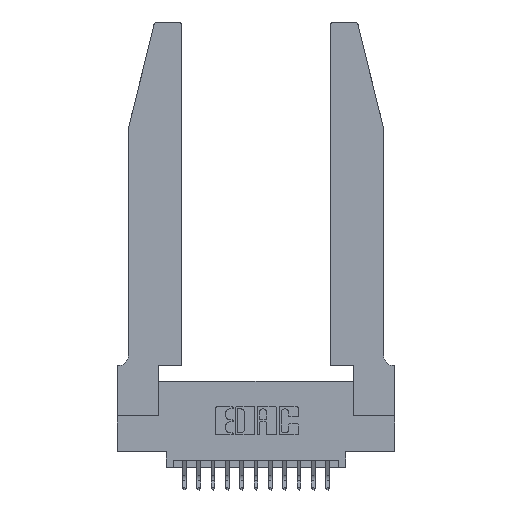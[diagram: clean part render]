
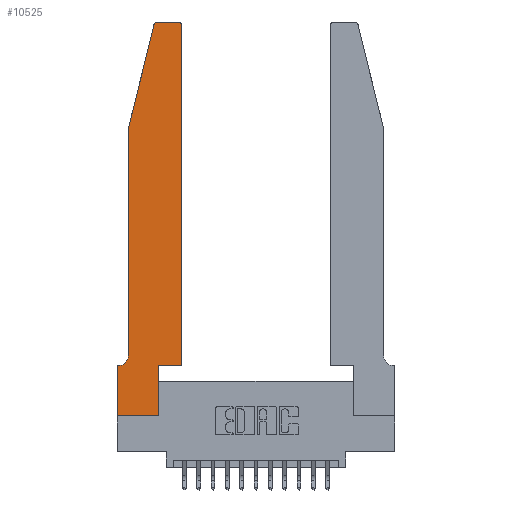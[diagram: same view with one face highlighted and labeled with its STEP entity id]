
A CAD part, top view. The second image highlights one B-rep face of the part: STEP entity #10525.
In plain terms, the highlighted planar face has unit normal (0, 0, 1).
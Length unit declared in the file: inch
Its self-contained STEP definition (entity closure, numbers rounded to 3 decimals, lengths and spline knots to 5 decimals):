
#69 = VERTEX_POINT ( 'NONE', #10907 ) ;
#88 = CARTESIAN_POINT ( 'NONE',  ( 0.2865, 0.35, 0.37 ) ) ;
#146 = VERTEX_POINT ( 'NONE', #14226 ) ;
#669 = ORIENTED_EDGE ( 'NONE', *, *, #8839, .T. ) ;
#888 = VERTEX_POINT ( 'NONE', #4528 ) ;
#901 = VECTOR ( 'NONE', #5757, 39.37008 ) ;
#990 = LINE ( 'NONE', #12985, #11191 ) ;
#1097 = CARTESIAN_POINT ( 'NONE',  ( 0.0755, 2., 0.37 ) ) ;
#1252 = VERTEX_POINT ( 'NONE', #10823 ) ;
#1785 = ORIENTED_EDGE ( 'NONE', *, *, #10338, .T. ) ;
#1799 = CARTESIAN_POINT ( 'NONE',  ( 0.4505, 0.35, 0.37 ) ) ;
#1834 = DIRECTION ( 'NONE',  ( -0.239, -0.971, 0. ) ) ;
#1997 = AXIS2_PLACEMENT_3D ( 'NONE', #11527, #16933, #4441 ) ;
#2156 = VERTEX_POINT ( 'NONE', #88 ) ;
#2163 = CIRCLE ( 'NONE', #17287, 0.03 ) ;
#2336 = CIRCLE ( 'NONE', #3263, 0.03 ) ;
#2740 = VERTEX_POINT ( 'NONE', #17051 ) ;
#2990 = VERTEX_POINT ( 'NONE', #9995 ) ;
#3242 = CARTESIAN_POINT ( 'NONE',  ( 0.4205, 2.72, 0.37 ) ) ;
#3263 = AXIS2_PLACEMENT_3D ( 'NONE', #3242, #10271, #14206 ) ;
#3358 = EDGE_CURVE ( 'NONE', #2156, #6280, #3509, .T. ) ;
#3509 = LINE ( 'NONE', #16581, #901 ) ;
#3695 = VECTOR ( 'NONE', #15009, 39.37008 ) ;
#3942 = LINE ( 'NONE', #11703, #5666 ) ;
#4131 = VECTOR ( 'NONE', #14072, 39.37008 ) ;
#4154 = VERTEX_POINT ( 'NONE', #14728 ) ;
#4338 = EDGE_CURVE ( 'NONE', #12381, #4154, #16650, .T. ) ;
#4441 = DIRECTION ( 'NONE',  ( 1., 0., 0. ) ) ;
#4528 = CARTESIAN_POINT ( 'NONE',  ( 0.4505, 2.72, 0.37 ) ) ;
#4531 = ORIENTED_EDGE ( 'NONE', *, *, #3358, .T. ) ;
#4559 = VECTOR ( 'NONE', #6593, 39.37008 ) ;
#4934 = FACE_OUTER_BOUND ( 'NONE', #13743, .T. ) ;
#5195 = DIRECTION ( 'NONE',  ( 1., 0., 0. ) ) ;
#5666 = VECTOR ( 'NONE', #7370, 39.37008 ) ;
#5748 = VERTEX_POINT ( 'NONE', #17686 ) ;
#5757 = DIRECTION ( 'NONE',  ( 1., 0., 0. ) ) ;
#5885 = VECTOR ( 'NONE', #16787, 39.37008 ) ;
#5897 = CARTESIAN_POINT ( 'NONE',  ( 0., 0., 0.37 ) ) ;
#6048 = ORIENTED_EDGE ( 'NONE', *, *, #14073, .T. ) ;
#6151 = ORIENTED_EDGE ( 'NONE', *, *, #4338, .T. ) ;
#6232 = EDGE_CURVE ( 'NONE', #6280, #888, #11156, .T. ) ;
#6280 = VERTEX_POINT ( 'NONE', #1799 ) ;
#6593 = DIRECTION ( 'NONE',  ( -1., 0., 0. ) ) ;
#6713 = LINE ( 'NONE', #16643, #4131 ) ;
#6915 = LINE ( 'NONE', #12071, #4559 ) ;
#7370 = DIRECTION ( 'NONE',  ( 0., -1., 0. ) ) ;
#7428 = EDGE_CURVE ( 'NONE', #2990, #14704, #3942, .T. ) ;
#7448 = VECTOR ( 'NONE', #14444, 39.37008 ) ;
#8438 = LINE ( 'NONE', #1097, #3695 ) ;
#8839 = EDGE_CURVE ( 'NONE', #69, #2740, #6915, .T. ) ;
#9248 = ORIENTED_EDGE ( 'NONE', *, *, #6232, .T. ) ;
#9437 = ORIENTED_EDGE ( 'NONE', *, *, #16857, .T. ) ;
#9463 = DIRECTION ( 'NONE',  ( -1., 0., 0. ) ) ;
#9907 = LINE ( 'NONE', #15202, #17660 ) ;
#9995 = CARTESIAN_POINT ( 'NONE',  ( 0., 0.35, 0.37 ) ) ;
#10022 = EDGE_CURVE ( 'NONE', #888, #69, #2336, .T. ) ;
#10271 = DIRECTION ( 'NONE',  ( 0., 0., 1. ) ) ;
#10294 = ORIENTED_EDGE ( 'NONE', *, *, #13024, .T. ) ;
#10338 = EDGE_CURVE ( 'NONE', #5748, #2156, #9907, .T. ) ;
#10525 = ADVANCED_FACE ( 'NONE', ( #4934 ), #14184, .T. ) ;
#10802 = CARTESIAN_POINT ( 'NONE',  ( 0.0055, 0.42, 0.37 ) ) ;
#10823 = CARTESIAN_POINT ( 'NONE',  ( 0.0755, 2., 0.37 ) ) ;
#10907 = CARTESIAN_POINT ( 'NONE',  ( 0.4205, 2.75, 0.37 ) ) ;
#11156 = LINE ( 'NONE', #11497, #7448 ) ;
#11191 = VECTOR ( 'NONE', #1834, 39.37008 ) ;
#11497 = CARTESIAN_POINT ( 'NONE',  ( 0.4505, 0.35, 0.37 ) ) ;
#11527 = CARTESIAN_POINT ( 'NONE',  ( 0., 0.35, 0.37 ) ) ;
#11654 = AXIS2_PLACEMENT_3D ( 'NONE', #10802, #12273, #9463 ) ;
#11703 = CARTESIAN_POINT ( 'NONE',  ( 0., 0., 0.37 ) ) ;
#12071 = CARTESIAN_POINT ( 'NONE',  ( 0.2605, 2.75, 0.37 ) ) ;
#12251 = CARTESIAN_POINT ( 'NONE',  ( 0.0755, 0.42, 0.37 ) ) ;
#12273 = DIRECTION ( 'NONE',  ( 0., 0., -1. ) ) ;
#12381 = VERTEX_POINT ( 'NONE', #12251 ) ;
#12383 = DIRECTION ( 'NONE',  ( 0., 1., 0. ) ) ;
#12413 = LINE ( 'NONE', #15237, #5885 ) ;
#12985 = CARTESIAN_POINT ( 'NONE',  ( 0.0755, 2., 0.37 ) ) ;
#13024 = EDGE_CURVE ( 'NONE', #4154, #2990, #12413, .T. ) ;
#13469 = ORIENTED_EDGE ( 'NONE', *, *, #13664, .T. ) ;
#13623 = CARTESIAN_POINT ( 'NONE',  ( 0.284, 2.72, 0.37 ) ) ;
#13664 = EDGE_CURVE ( 'NONE', #14704, #5748, #6713, .T. ) ;
#13743 = EDGE_LOOP ( 'NONE', ( #669, #6048, #9437, #14114, #6151, #10294, #14090, #13469, #1785, #4531, #9248, #16974 ) ) ;
#14072 = DIRECTION ( 'NONE',  ( 1., 0., 0. ) ) ;
#14073 = EDGE_CURVE ( 'NONE', #2740, #146, #2163, .T. ) ;
#14087 = EDGE_CURVE ( 'NONE', #1252, #12381, #8438, .T. ) ;
#14090 = ORIENTED_EDGE ( 'NONE', *, *, #7428, .T. ) ;
#14114 = ORIENTED_EDGE ( 'NONE', *, *, #14087, .T. ) ;
#14184 = PLANE ( 'NONE',  #1997 ) ;
#14206 = DIRECTION ( 'NONE',  ( 1., 0., 0. ) ) ;
#14226 = CARTESIAN_POINT ( 'NONE',  ( 0.25487, 2.72718, 0.37 ) ) ;
#14444 = DIRECTION ( 'NONE',  ( 0., 1., 0. ) ) ;
#14704 = VERTEX_POINT ( 'NONE', #5897 ) ;
#14728 = CARTESIAN_POINT ( 'NONE',  ( 0.0055, 0.35, 0.37 ) ) ;
#15009 = DIRECTION ( 'NONE',  ( 0., -1., 0. ) ) ;
#15202 = CARTESIAN_POINT ( 'NONE',  ( 0.2865, 0.35, 0.37 ) ) ;
#15237 = CARTESIAN_POINT ( 'NONE',  ( 0.0755, 0.35, 0.37 ) ) ;
#16581 = CARTESIAN_POINT ( 'NONE',  ( 0.4505, 0.35, 0.37 ) ) ;
#16643 = CARTESIAN_POINT ( 'NONE',  ( 0., 0., 0.37 ) ) ;
#16650 = CIRCLE ( 'NONE', #11654, 0.07 ) ;
#16787 = DIRECTION ( 'NONE',  ( -1., 0., 0. ) ) ;
#16857 = EDGE_CURVE ( 'NONE', #146, #1252, #990, .T. ) ;
#16933 = DIRECTION ( 'NONE',  ( 0., 0., 1. ) ) ;
#16974 = ORIENTED_EDGE ( 'NONE', *, *, #10022, .T. ) ;
#17051 = CARTESIAN_POINT ( 'NONE',  ( 0.284, 2.75, 0.37 ) ) ;
#17287 = AXIS2_PLACEMENT_3D ( 'NONE', #13623, #17702, #5195 ) ;
#17660 = VECTOR ( 'NONE', #12383, 39.37008 ) ;
#17686 = CARTESIAN_POINT ( 'NONE',  ( 0.2865, 0., 0.37 ) ) ;
#17702 = DIRECTION ( 'NONE',  ( 0., 0., 1. ) ) ;
